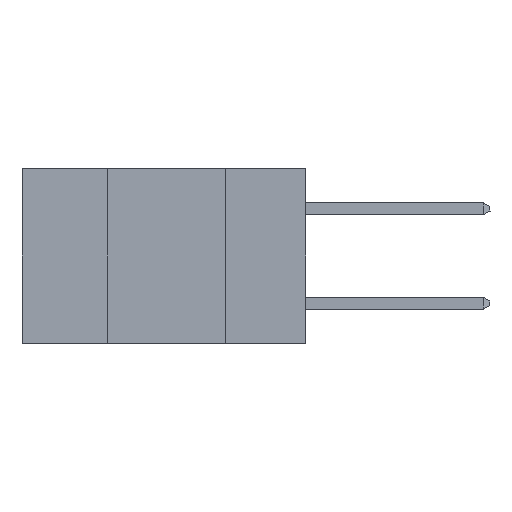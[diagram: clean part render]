
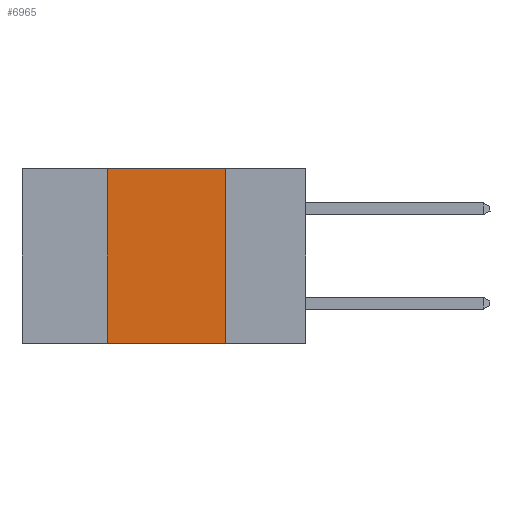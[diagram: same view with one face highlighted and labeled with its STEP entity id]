
A CAD part, left-side view. The second image highlights one B-rep face of the part: STEP entity #6965.
In plain terms, the highlighted planar face has unit normal (-1, 0, 0).
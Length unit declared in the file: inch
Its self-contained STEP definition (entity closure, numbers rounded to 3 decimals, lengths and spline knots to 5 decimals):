
#119 = DIRECTION ( 'NONE',  ( 0., 0., -1. ) ) ;
#231 = VERTEX_POINT ( 'NONE', #4826 ) ;
#505 = EDGE_CURVE ( 'NONE', #231, #2405, #5186, .T. ) ;
#1171 = DIRECTION ( 'NONE',  ( 0., -1., 0. ) ) ;
#1246 = FACE_OUTER_BOUND ( 'NONE', #5767, .T. ) ;
#1617 = VECTOR ( 'NONE', #4707, 39.37008 ) ;
#2405 = VERTEX_POINT ( 'NONE', #3271 ) ;
#3271 = CARTESIAN_POINT ( 'NONE',  ( 0., 0.42, 0. ) ) ;
#3505 = DIRECTION ( 'NONE',  ( 0., 0., -1. ) ) ;
#3725 = ORIENTED_EDGE ( 'NONE', *, *, #505, .F. ) ;
#3756 = CARTESIAN_POINT ( 'NONE',  ( 0., 0.6, 0. ) ) ;
#4325 = ORIENTED_EDGE ( 'NONE', *, *, #6239, .T. ) ;
#4402 = VECTOR ( 'NONE', #7536, 39.37008 ) ;
#4707 = DIRECTION ( 'NONE',  ( 0., 0., 1. ) ) ;
#4826 = CARTESIAN_POINT ( 'NONE',  ( 0., 0.42, -0.37 ) ) ;
#5040 = EDGE_CURVE ( 'NONE', #6011, #5832, #6818, .T. ) ;
#5154 = PLANE ( 'NONE',  #5641 ) ;
#5186 = LINE ( 'NONE', #5252, #1617 ) ;
#5252 = CARTESIAN_POINT ( 'NONE',  ( 0., 0.42, 0. ) ) ;
#5336 = CARTESIAN_POINT ( 'NONE',  ( 0., 0.6, -0.37 ) ) ;
#5596 = DIRECTION ( 'NONE',  ( 1., 0., 0. ) ) ;
#5641 = AXIS2_PLACEMENT_3D ( 'NONE', #3756, #5596, #3505 ) ;
#5644 = ORIENTED_EDGE ( 'NONE', *, *, #5040, .F. ) ;
#5702 = CARTESIAN_POINT ( 'NONE',  ( 0., 0.17, -0.37 ) ) ;
#5767 = EDGE_LOOP ( 'NONE', ( #5644, #8631, #3725, #4325 ) ) ;
#5832 = VERTEX_POINT ( 'NONE', #5702 ) ;
#5914 = CARTESIAN_POINT ( 'NONE',  ( 0., 0.17, 0. ) ) ;
#6011 = VERTEX_POINT ( 'NONE', #8771 ) ;
#6239 = EDGE_CURVE ( 'NONE', #231, #5832, #9151, .T. ) ;
#6720 = LINE ( 'NONE', #7703, #7400 ) ;
#6818 = LINE ( 'NONE', #5914, #8076 ) ;
#6965 = ADVANCED_FACE ( 'NONE', ( #1246 ), #5154, .F. ) ;
#7221 = EDGE_CURVE ( 'NONE', #2405, #6011, #6720, .T. ) ;
#7400 = VECTOR ( 'NONE', #1171, 39.37008 ) ;
#7536 = DIRECTION ( 'NONE',  ( 0., -1., 0. ) ) ;
#7703 = CARTESIAN_POINT ( 'NONE',  ( 0., 0.6, 0. ) ) ;
#8076 = VECTOR ( 'NONE', #119, 39.37008 ) ;
#8631 = ORIENTED_EDGE ( 'NONE', *, *, #7221, .F. ) ;
#8771 = CARTESIAN_POINT ( 'NONE',  ( 0., 0.17, 0. ) ) ;
#9151 = LINE ( 'NONE', #5336, #4402 ) ;
